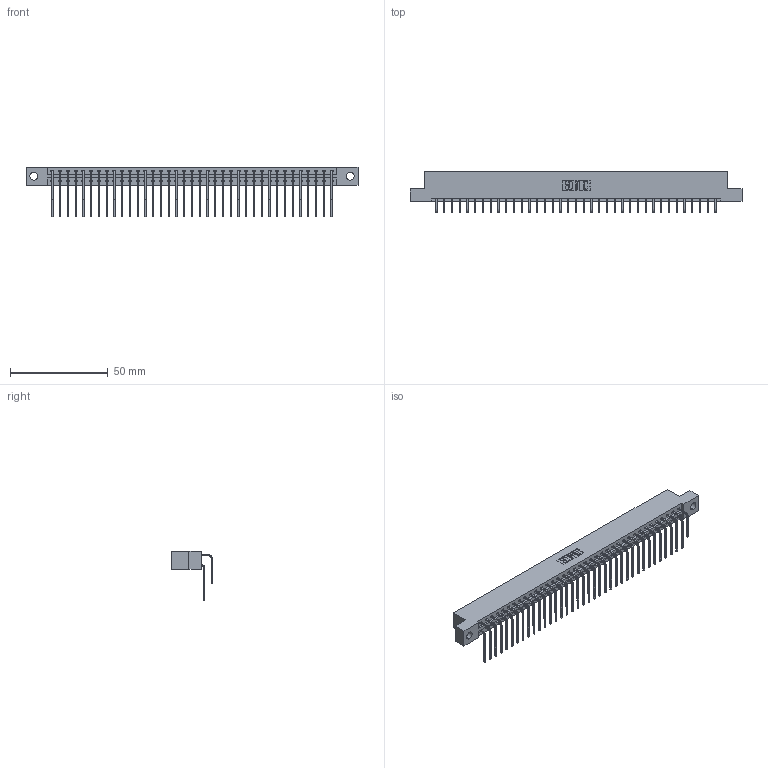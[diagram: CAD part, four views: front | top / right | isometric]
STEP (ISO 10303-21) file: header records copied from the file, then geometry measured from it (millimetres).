
FILE_DESCRIPTION (( 'STEP AP203' ), '1' );
FILE_NAME ('337-074-559-204.STEP', '2018-08-11T18:37:17', ( '' ), ( '' ), 'SwSTEP 2.0', 'SolidWorks 2016', '' );
FILE_SCHEMA (( 'CONFIG_CONTROL_DESIGN' ));
Length unit declared in the file: inch
Products named in the file (4): 345-292-001_559 Tail - 2; 337-074-559-204; 337 Part_Flush Mounting Lugs - 0.156 Dia-TH; 345-292-001_558 559 Tail - 1
Assembly tree (75 placements, depth 2):
  337-074-559-204
    337 Part_Flush Mounting Lugs - 0.156 Dia-TH
    345-292-001_558 559 Tail - 1  x37
    345-292-001_559 Tail - 2  x37
Bounding box: 169.62 x 20.9 x 25.53 mm (x, y, z)
Volume: 18148.5 mm3; surface area: 22409.2 mm2
Topology: 75 solids, 75 shells, 4258 faces, 12669 edges, 8346 vertices
Faces by surface type: plane 3030, cylinder 1228
Entity records: 31121 total; most frequent: CARTESIAN_POINT 5293, ORIENTED_EDGE 5178, DIRECTION 4493, EDGE_CURVE 2589, LINE 2421, VECTOR 2421, VERTEX_POINT 1722, AXIS2_PLACEMENT_3D 1036
